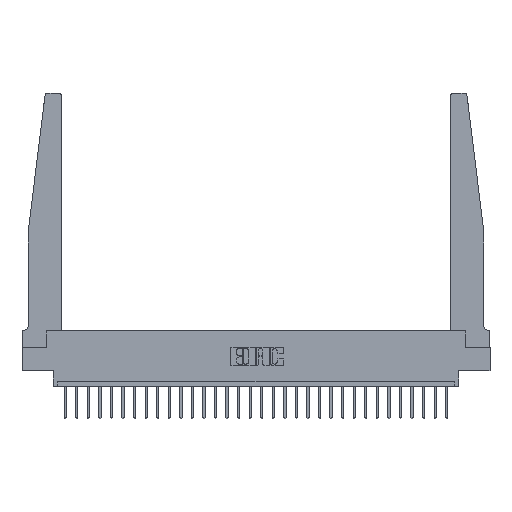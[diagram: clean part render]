
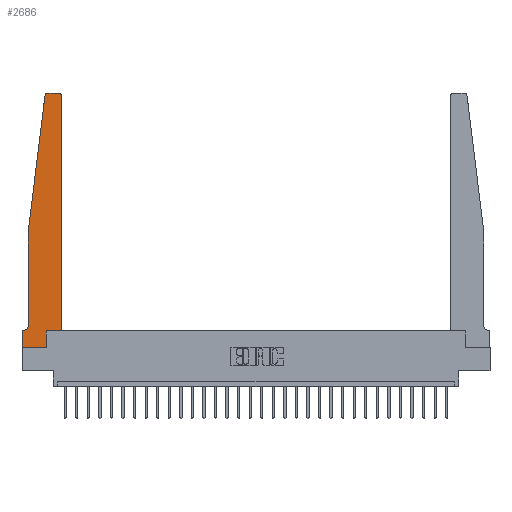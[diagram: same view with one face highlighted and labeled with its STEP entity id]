
A CAD part, top view. The second image highlights one B-rep face of the part: STEP entity #2686.
In plain terms, the highlighted planar face has unit normal (0, 0, 1).
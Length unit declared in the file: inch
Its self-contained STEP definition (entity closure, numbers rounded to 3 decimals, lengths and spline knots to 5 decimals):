
#25 = DIRECTION ( 'NONE',  ( 0., 1., 0. ) ) ;
#92 = ORIENTED_EDGE ( 'NONE', *, *, #2136, .T. ) ;
#221 = DIRECTION ( 'NONE',  ( 1., 0., 0. ) ) ;
#542 = ORIENTED_EDGE ( 'NONE', *, *, #4087, .T. ) ;
#751 = VECTOR ( 'NONE', #25, 39.37008 ) ;
#926 = ORIENTED_EDGE ( 'NONE', *, *, #2264, .T. ) ;
#1220 = DIRECTION ( 'NONE',  ( -1., 0., 0. ) ) ;
#1837 = VERTEX_POINT ( 'NONE', #22589 ) ;
#1852 = CARTESIAN_POINT ( 'NONE',  ( 0., 0., 0.37 ) ) ;
#1954 = CARTESIAN_POINT ( 'NONE',  ( 0.2605, 0.18, 0.37 ) ) ;
#2136 = EDGE_CURVE ( 'NONE', #16602, #4241, #20036, .T. ) ;
#2264 = EDGE_CURVE ( 'NONE', #9343, #16311, #20669, .T. ) ;
#2429 = DIRECTION ( 'NONE',  ( 1., 0., 0. ) ) ;
#2494 = EDGE_CURVE ( 'NONE', #7391, #26260, #7265, .T. ) ;
#2646 = VERTEX_POINT ( 'NONE', #12643 ) ;
#2686 = ADVANCED_FACE ( 'NONE', ( #21305 ), #7291, .T. ) ;
#3636 = ORIENTED_EDGE ( 'NONE', *, *, #18636, .T. ) ;
#3806 = CARTESIAN_POINT ( 'NONE',  ( 0.425, 0.18, 0.37 ) ) ;
#3877 = VECTOR ( 'NONE', #3960, 39.37008 ) ;
#3960 = DIRECTION ( 'NONE',  ( 0., -1., 0. ) ) ;
#4087 = EDGE_CURVE ( 'NONE', #4241, #5209, #12703, .T. ) ;
#4170 = ORIENTED_EDGE ( 'NONE', *, *, #22724, .T. ) ;
#4241 = VERTEX_POINT ( 'NONE', #25283 ) ;
#4858 = EDGE_LOOP ( 'NONE', ( #4170, #20825, #6783, #15027, #22027, #3636, #26684, #24118, #926, #25131, #92, #542 ) ) ;
#5209 = VERTEX_POINT ( 'NONE', #7154 ) ;
#6285 = DIRECTION ( 'NONE',  ( 1., 0., 0. ) ) ;
#6552 = DIRECTION ( 'NONE',  ( 0., 0., 1. ) ) ;
#6617 = EDGE_CURVE ( 'NONE', #16311, #16602, #10246, .T. ) ;
#6783 = ORIENTED_EDGE ( 'NONE', *, *, #17289, .T. ) ;
#7154 = CARTESIAN_POINT ( 'NONE',  ( 0.395, 2.75, 0.37 ) ) ;
#7229 = LINE ( 'NONE', #21640, #18665 ) ;
#7265 = CIRCLE ( 'NONE', #19670, 0.05 ) ;
#7291 = PLANE ( 'NONE',  #12656 ) ;
#7391 = VERTEX_POINT ( 'NONE', #26330 ) ;
#8457 = DIRECTION ( 'NONE',  ( 0., -1., 0. ) ) ;
#8524 = DIRECTION ( 'NONE',  ( 0., 1., 0. ) ) ;
#8694 = EDGE_CURVE ( 'NONE', #25117, #12427, #21905, .T. ) ;
#8981 = CARTESIAN_POINT ( 'NONE',  ( 0.2605, 0., 0.37 ) ) ;
#9343 = VERTEX_POINT ( 'NONE', #8981 ) ;
#9773 = DIRECTION ( 'NONE',  ( 1., 0., 0. ) ) ;
#9838 = CARTESIAN_POINT ( 'NONE',  ( 0.24675, 2.72367, 0.37 ) ) ;
#10220 = VECTOR ( 'NONE', #22652, 39.37008 ) ;
#10246 = LINE ( 'NONE', #12624, #23012 ) ;
#12112 = CARTESIAN_POINT ( 'NONE',  ( 0., 0., 0.37 ) ) ;
#12427 = VERTEX_POINT ( 'NONE', #9838 ) ;
#12624 = CARTESIAN_POINT ( 'NONE',  ( 0.425, 0.18, 0.37 ) ) ;
#12643 = CARTESIAN_POINT ( 'NONE',  ( 0., 0.1875, 0.37 ) ) ;
#12656 = AXIS2_PLACEMENT_3D ( 'NONE', #17798, #24148, #9773 ) ;
#12703 = CIRCLE ( 'NONE', #26396, 0.03 ) ;
#13633 = DIRECTION ( 'NONE',  ( 0., 0., -1. ) ) ;
#13953 = LINE ( 'NONE', #19940, #22489 ) ;
#14434 = VECTOR ( 'NONE', #8524, 39.37008 ) ;
#14758 = CARTESIAN_POINT ( 'NONE',  ( 0.395, 2.72, 0.37 ) ) ;
#15027 = ORIENTED_EDGE ( 'NONE', *, *, #19607, .T. ) ;
#15180 = VECTOR ( 'NONE', #8457, 39.37008 ) ;
#15297 = CARTESIAN_POINT ( 'NONE',  ( 0.27653, 2.72, 0.37 ) ) ;
#15548 = LINE ( 'NONE', #23395, #15180 ) ;
#16311 = VERTEX_POINT ( 'NONE', #25810 ) ;
#16602 = VERTEX_POINT ( 'NONE', #3806 ) ;
#16953 = VECTOR ( 'NONE', #20318, 39.37008 ) ;
#17289 = EDGE_CURVE ( 'NONE', #12427, #27004, #22878, .T. ) ;
#17798 = CARTESIAN_POINT ( 'NONE',  ( 0., 0.1875, 0.37 ) ) ;
#17844 = CARTESIAN_POINT ( 'NONE',  ( 0.065, 1.25, 0.37 ) ) ;
#18053 = CARTESIAN_POINT ( 'NONE',  ( 0.015, 0.1875, 0.37 ) ) ;
#18582 = CARTESIAN_POINT ( 'NONE',  ( 0.065, 1.25, 0.37 ) ) ;
#18636 = EDGE_CURVE ( 'NONE', #26260, #2646, #13953, .T. ) ;
#18665 = VECTOR ( 'NONE', #19606, 39.37008 ) ;
#19606 = DIRECTION ( 'NONE',  ( -1., 0., 0. ) ) ;
#19607 = EDGE_CURVE ( 'NONE', #27004, #7391, #15548, .T. ) ;
#19670 = AXIS2_PLACEMENT_3D ( 'NONE', #24277, #13633, #1220 ) ;
#19940 = CARTESIAN_POINT ( 'NONE',  ( 0.065, 0.1875, 0.37 ) ) ;
#20036 = LINE ( 'NONE', #22804, #751 ) ;
#20042 = CARTESIAN_POINT ( 'NONE',  ( 0.27653, 2.75, 0.37 ) ) ;
#20209 = DIRECTION ( 'NONE',  ( -1., 0., 0. ) ) ;
#20318 = DIRECTION ( 'NONE',  ( -0.122, -0.992, 0. ) ) ;
#20669 = LINE ( 'NONE', #1954, #14434 ) ;
#20825 = ORIENTED_EDGE ( 'NONE', *, *, #8694, .T. ) ;
#21305 = FACE_OUTER_BOUND ( 'NONE', #4858, .T. ) ;
#21446 = DIRECTION ( 'NONE',  ( 0., 0., 1. ) ) ;
#21640 = CARTESIAN_POINT ( 'NONE',  ( 0.25, 2.75, 0.37 ) ) ;
#21905 = CIRCLE ( 'NONE', #24353, 0.03 ) ;
#22027 = ORIENTED_EDGE ( 'NONE', *, *, #2494, .T. ) ;
#22221 = LINE ( 'NONE', #1852, #3877 ) ;
#22489 = VECTOR ( 'NONE', #20209, 39.37008 ) ;
#22589 = CARTESIAN_POINT ( 'NONE',  ( 0., 0., 0.37 ) ) ;
#22652 = DIRECTION ( 'NONE',  ( 1., 0., 0. ) ) ;
#22724 = EDGE_CURVE ( 'NONE', #5209, #25117, #7229, .T. ) ;
#22804 = CARTESIAN_POINT ( 'NONE',  ( 0.425, 0.18, 0.37 ) ) ;
#22878 = LINE ( 'NONE', #18582, #16953 ) ;
#23012 = VECTOR ( 'NONE', #221, 39.37008 ) ;
#23395 = CARTESIAN_POINT ( 'NONE',  ( 0.065, 1.25, 0.37 ) ) ;
#23644 = LINE ( 'NONE', #12112, #10220 ) ;
#24118 = ORIENTED_EDGE ( 'NONE', *, *, #24636, .T. ) ;
#24148 = DIRECTION ( 'NONE',  ( 0., 0., 1. ) ) ;
#24277 = CARTESIAN_POINT ( 'NONE',  ( 0.015, 0.2375, 0.37 ) ) ;
#24353 = AXIS2_PLACEMENT_3D ( 'NONE', #15297, #21446, #2429 ) ;
#24636 = EDGE_CURVE ( 'NONE', #1837, #9343, #23644, .T. ) ;
#25117 = VERTEX_POINT ( 'NONE', #20042 ) ;
#25131 = ORIENTED_EDGE ( 'NONE', *, *, #6617, .T. ) ;
#25283 = CARTESIAN_POINT ( 'NONE',  ( 0.425, 2.72, 0.37 ) ) ;
#25810 = CARTESIAN_POINT ( 'NONE',  ( 0.2605, 0.18, 0.37 ) ) ;
#26260 = VERTEX_POINT ( 'NONE', #18053 ) ;
#26330 = CARTESIAN_POINT ( 'NONE',  ( 0.065, 0.2375, 0.37 ) ) ;
#26396 = AXIS2_PLACEMENT_3D ( 'NONE', #14758, #6552, #6285 ) ;
#26684 = ORIENTED_EDGE ( 'NONE', *, *, #26965, .T. ) ;
#26965 = EDGE_CURVE ( 'NONE', #2646, #1837, #22221, .T. ) ;
#27004 = VERTEX_POINT ( 'NONE', #17844 ) ;
